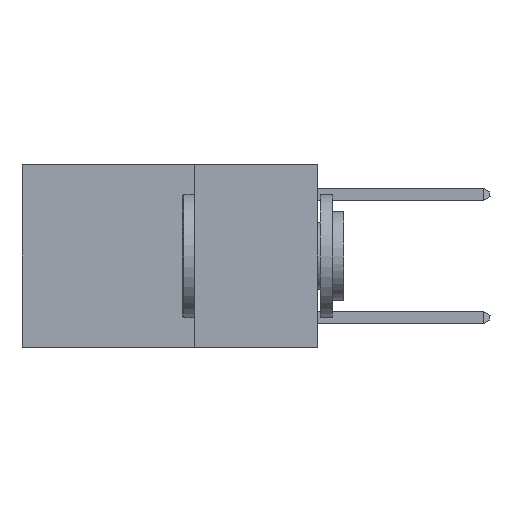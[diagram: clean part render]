
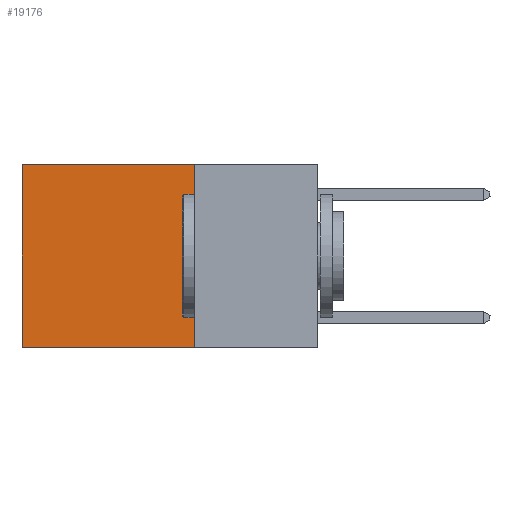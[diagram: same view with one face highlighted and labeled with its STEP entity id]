
A CAD part, left-side view. The second image highlights one B-rep face of the part: STEP entity #19176.
In plain terms, the highlighted planar face has unit normal (-1, 0, 0).
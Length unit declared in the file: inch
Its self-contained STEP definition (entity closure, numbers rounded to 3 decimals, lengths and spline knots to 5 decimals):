
#1737 = DIRECTION ( 'NONE',  ( 0., 0., -1. ) ) ;
#1952 = FACE_OUTER_BOUND ( 'NONE', #18949, .T. ) ;
#3931 = CARTESIAN_POINT ( 'NONE',  ( 0.2625, 0.6, 0. ) ) ;
#4155 = VERTEX_POINT ( 'NONE', #20057 ) ;
#4679 = ORIENTED_EDGE ( 'NONE', *, *, #15636, .T. ) ;
#5324 = CARTESIAN_POINT ( 'NONE',  ( 0.2625, 0.25, -0.37 ) ) ;
#5363 = ORIENTED_EDGE ( 'NONE', *, *, #15517, .F. ) ;
#5604 = DIRECTION ( 'NONE',  ( 0., 0., -1. ) ) ;
#5655 = DIRECTION ( 'NONE',  ( 0., 1., 0. ) ) ;
#6689 = EDGE_CURVE ( 'NONE', #11413, #16768, #16585, .T. ) ;
#9047 = AXIS2_PLACEMENT_3D ( 'NONE', #15238, #17217, #1737 ) ;
#9425 = LINE ( 'NONE', #20880, #12902 ) ;
#10562 = VERTEX_POINT ( 'NONE', #14442 ) ;
#10764 = VECTOR ( 'NONE', #18743, 39.37008 ) ;
#11019 = CARTESIAN_POINT ( 'NONE',  ( 0.2625, 0.25, 0. ) ) ;
#11413 = VERTEX_POINT ( 'NONE', #11019 ) ;
#12902 = VECTOR ( 'NONE', #5655, 39.37008 ) ;
#12970 = LINE ( 'NONE', #21760, #10764 ) ;
#13273 = VECTOR ( 'NONE', #20103, 39.37008 ) ;
#14442 = CARTESIAN_POINT ( 'NONE',  ( 0.2625, 0.6, -0.37 ) ) ;
#15238 = CARTESIAN_POINT ( 'NONE',  ( 0.2625, 0.25, 0. ) ) ;
#15301 = VECTOR ( 'NONE', #5604, 39.37008 ) ;
#15517 = EDGE_CURVE ( 'NONE', #16768, #10562, #9425, .T. ) ;
#15550 = LINE ( 'NONE', #3931, #15301 ) ;
#15636 = EDGE_CURVE ( 'NONE', #11413, #4155, #12970, .T. ) ;
#15763 = ORIENTED_EDGE ( 'NONE', *, *, #15912, .T. ) ;
#15912 = EDGE_CURVE ( 'NONE', #4155, #10562, #15550, .T. ) ;
#16585 = LINE ( 'NONE', #21656, #13273 ) ;
#16768 = VERTEX_POINT ( 'NONE', #5324 ) ;
#17217 = DIRECTION ( 'NONE',  ( 1., 0., 0. ) ) ;
#18743 = DIRECTION ( 'NONE',  ( 0., 1., 0. ) ) ;
#18871 = PLANE ( 'NONE',  #9047 ) ;
#18949 = EDGE_LOOP ( 'NONE', ( #15763, #5363, #20083, #4679 ) ) ;
#19176 = ADVANCED_FACE ( 'NONE', ( #1952 ), #18871, .F. ) ;
#20057 = CARTESIAN_POINT ( 'NONE',  ( 0.2625, 0.6, 0. ) ) ;
#20083 = ORIENTED_EDGE ( 'NONE', *, *, #6689, .F. ) ;
#20103 = DIRECTION ( 'NONE',  ( 0., 0., -1. ) ) ;
#20880 = CARTESIAN_POINT ( 'NONE',  ( 0.2625, 0.25, -0.37 ) ) ;
#21656 = CARTESIAN_POINT ( 'NONE',  ( 0.2625, 0.25, 0. ) ) ;
#21760 = CARTESIAN_POINT ( 'NONE',  ( 0.2625, 0.25, 0. ) ) ;
